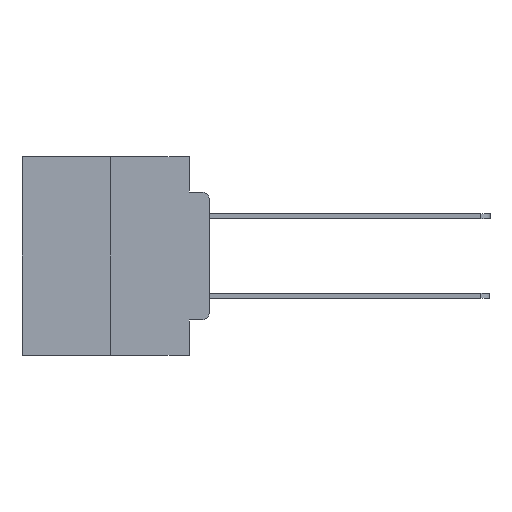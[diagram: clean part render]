
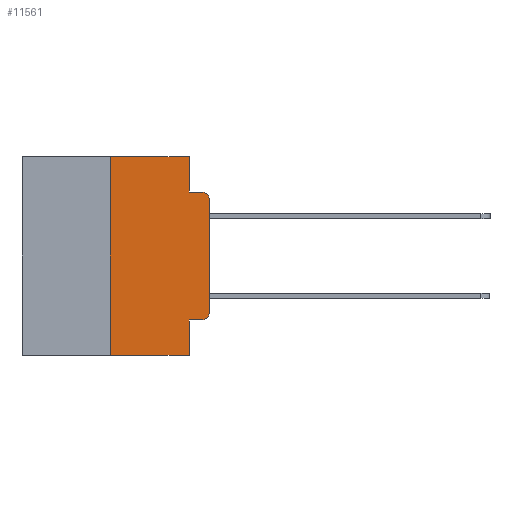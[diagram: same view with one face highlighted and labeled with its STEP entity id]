
A CAD part, left-side view. The second image highlights one B-rep face of the part: STEP entity #11561.
In plain terms, the highlighted planar face has unit normal (-1, 0, 0).
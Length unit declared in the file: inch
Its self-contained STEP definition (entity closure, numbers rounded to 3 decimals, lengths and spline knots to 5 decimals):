
#27 = FACE_OUTER_BOUND ( 'NONE', #21769, .T. ) ;
#985 = EDGE_CURVE ( 'NONE', #20791, #20087, #12282, .T. ) ;
#1033 = CARTESIAN_POINT ( 'NONE',  ( 0., 0.02, -0.4115 ) ) ;
#1753 = CARTESIAN_POINT ( 'NONE',  ( 0., 0.051, -0.5 ) ) ;
#1771 = VERTEX_POINT ( 'NONE', #8321 ) ;
#2288 = VECTOR ( 'NONE', #7016, 39.37008 ) ;
#2465 = EDGE_CURVE ( 'NONE', #23554, #1771, #26870, .T. ) ;
#4238 = ORIENTED_EDGE ( 'NONE', *, *, #985, .T. ) ;
#4433 = ORIENTED_EDGE ( 'NONE', *, *, #24224, .T. ) ;
#4512 = ORIENTED_EDGE ( 'NONE', *, *, #5417, .F. ) ;
#4574 = VERTEX_POINT ( 'NONE', #1033 ) ;
#4659 = PLANE ( 'NONE',  #10863 ) ;
#4735 = ORIENTED_EDGE ( 'NONE', *, *, #2465, .F. ) ;
#4775 = VECTOR ( 'NONE', #23188, 39.37008 ) ;
#4847 = ORIENTED_EDGE ( 'NONE', *, *, #27138, .F. ) ;
#5417 = EDGE_CURVE ( 'NONE', #1771, #20004, #7111, .T. ) ;
#5973 = EDGE_CURVE ( 'NONE', #9996, #19139, #15707, .T. ) ;
#5998 = LINE ( 'NONE', #18462, #22153 ) ;
#6233 = CIRCLE ( 'NONE', #20834, 0.02 ) ;
#6368 = CARTESIAN_POINT ( 'NONE',  ( 0., 0.051, -0.4115 ) ) ;
#6689 = VECTOR ( 'NONE', #9986, 39.37008 ) ;
#6799 = CARTESIAN_POINT ( 'NONE',  ( 0., 0.473, 0. ) ) ;
#7016 = DIRECTION ( 'NONE',  ( 0., -1., 0. ) ) ;
#7111 = LINE ( 'NONE', #25376, #17725 ) ;
#7371 = LINE ( 'NONE', #21768, #2288 ) ;
#7522 = CARTESIAN_POINT ( 'NONE',  ( 0., 0.25, -0.5 ) ) ;
#7669 = DIRECTION ( 'NONE',  ( 0., -1., 0. ) ) ;
#8129 = DIRECTION ( 'NONE',  ( -1., 0., 0. ) ) ;
#8199 = EDGE_CURVE ( 'NONE', #9996, #20957, #5998, .T. ) ;
#8321 = CARTESIAN_POINT ( 'NONE',  ( 0., 0.051, -0.0885 ) ) ;
#8711 = CARTESIAN_POINT ( 'NONE',  ( 0., 0., 0. ) ) ;
#8922 = ORIENTED_EDGE ( 'NONE', *, *, #8199, .F. ) ;
#9612 = VECTOR ( 'NONE', #12736, 39.37008 ) ;
#9986 = DIRECTION ( 'NONE',  ( 0., 0., 1. ) ) ;
#9996 = VERTEX_POINT ( 'NONE', #7522 ) ;
#10023 = VECTOR ( 'NONE', #27031, 39.37008 ) ;
#10383 = LINE ( 'NONE', #6368, #4775 ) ;
#10863 = AXIS2_PLACEMENT_3D ( 'NONE', #6799, #23598, #11038 ) ;
#10890 = VECTOR ( 'NONE', #26087, 39.37008 ) ;
#10937 = ORIENTED_EDGE ( 'NONE', *, *, #11951, .T. ) ;
#11038 = DIRECTION ( 'NONE',  ( 0., 0., -1. ) ) ;
#11061 = DIRECTION ( 'NONE',  ( -1., 0., 0. ) ) ;
#11101 = ORIENTED_EDGE ( 'NONE', *, *, #13923, .T. ) ;
#11561 = ADVANCED_FACE ( 'NONE', ( #27 ), #4659, .F. ) ;
#11951 = EDGE_CURVE ( 'NONE', #4574, #20791, #25219, .T. ) ;
#12282 = LINE ( 'NONE', #8711, #6689 ) ;
#12736 = DIRECTION ( 'NONE',  ( 0., 0., -1. ) ) ;
#13923 = EDGE_CURVE ( 'NONE', #23962, #4574, #10383, .T. ) ;
#14548 = CARTESIAN_POINT ( 'NONE',  ( 0., 0.473, -0.5 ) ) ;
#15707 = LINE ( 'NONE', #14548, #10023 ) ;
#16164 = CARTESIAN_POINT ( 'NONE',  ( 0., 0., -0.3915 ) ) ;
#17413 = ORIENTED_EDGE ( 'NONE', *, *, #5973, .T. ) ;
#17725 = VECTOR ( 'NONE', #7669, 39.37008 ) ;
#18462 = CARTESIAN_POINT ( 'NONE',  ( 0., 0.25, 0. ) ) ;
#18832 = CARTESIAN_POINT ( 'NONE',  ( 0., 0.25, 0. ) ) ;
#19139 = VERTEX_POINT ( 'NONE', #1753 ) ;
#19255 = CARTESIAN_POINT ( 'NONE',  ( 0., 0.051, 0. ) ) ;
#20004 = VERTEX_POINT ( 'NONE', #21957 ) ;
#20087 = VERTEX_POINT ( 'NONE', #20248 ) ;
#20248 = CARTESIAN_POINT ( 'NONE',  ( 0., 0., -0.1085 ) ) ;
#20271 = AXIS2_PLACEMENT_3D ( 'NONE', #20821, #8129, #22851 ) ;
#20572 = DIRECTION ( 'NONE',  ( 0., 0., 1. ) ) ;
#20791 = VERTEX_POINT ( 'NONE', #16164 ) ;
#20821 = CARTESIAN_POINT ( 'NONE',  ( 0., 0.02, -0.3915 ) ) ;
#20834 = AXIS2_PLACEMENT_3D ( 'NONE', #23615, #11061, #25661 ) ;
#20957 = VERTEX_POINT ( 'NONE', #18832 ) ;
#21121 = CARTESIAN_POINT ( 'NONE',  ( 0., 0.051, 0. ) ) ;
#21768 = CARTESIAN_POINT ( 'NONE',  ( 0., 0.473, 0. ) ) ;
#21769 = EDGE_LOOP ( 'NONE', ( #4238, #4433, #4512, #4735, #4847, #8922, #17413, #24992, #11101, #10937 ) ) ;
#21957 = CARTESIAN_POINT ( 'NONE',  ( 0., 0.02, -0.0885 ) ) ;
#22153 = VECTOR ( 'NONE', #20572, 39.37008 ) ;
#22353 = EDGE_CURVE ( 'NONE', #23962, #19139, #26313, .T. ) ;
#22851 = DIRECTION ( 'NONE',  ( 0., 0., -1. ) ) ;
#23188 = DIRECTION ( 'NONE',  ( 0., -1., 0. ) ) ;
#23554 = VERTEX_POINT ( 'NONE', #19255 ) ;
#23598 = DIRECTION ( 'NONE',  ( 1., 0., 0. ) ) ;
#23615 = CARTESIAN_POINT ( 'NONE',  ( 0., 0.02, -0.1085 ) ) ;
#23962 = VERTEX_POINT ( 'NONE', #24786 ) ;
#24224 = EDGE_CURVE ( 'NONE', #20087, #20004, #6233, .T. ) ;
#24786 = CARTESIAN_POINT ( 'NONE',  ( 0., 0.051, -0.4115 ) ) ;
#24992 = ORIENTED_EDGE ( 'NONE', *, *, #22353, .F. ) ;
#25219 = CIRCLE ( 'NONE', #20271, 0.02 ) ;
#25376 = CARTESIAN_POINT ( 'NONE',  ( 0., 0.051, -0.0885 ) ) ;
#25661 = DIRECTION ( 'NONE',  ( 0., 0., -1. ) ) ;
#26059 = CARTESIAN_POINT ( 'NONE',  ( 0., 0.051, 0. ) ) ;
#26087 = DIRECTION ( 'NONE',  ( 0., 0., -1. ) ) ;
#26313 = LINE ( 'NONE', #21121, #9612 ) ;
#26870 = LINE ( 'NONE', #26059, #10890 ) ;
#27031 = DIRECTION ( 'NONE',  ( 0., -1., 0. ) ) ;
#27138 = EDGE_CURVE ( 'NONE', #20957, #23554, #7371, .T. ) ;
